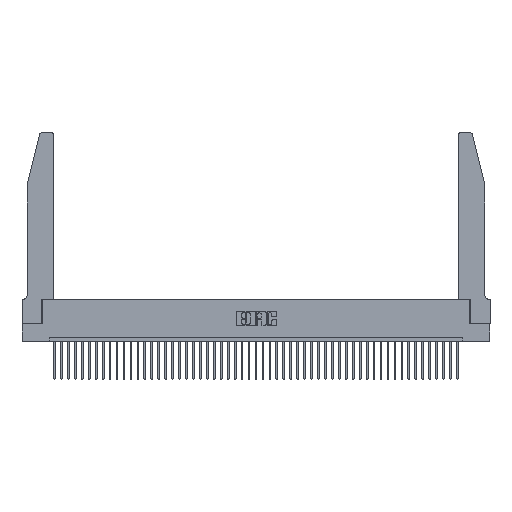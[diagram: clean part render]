
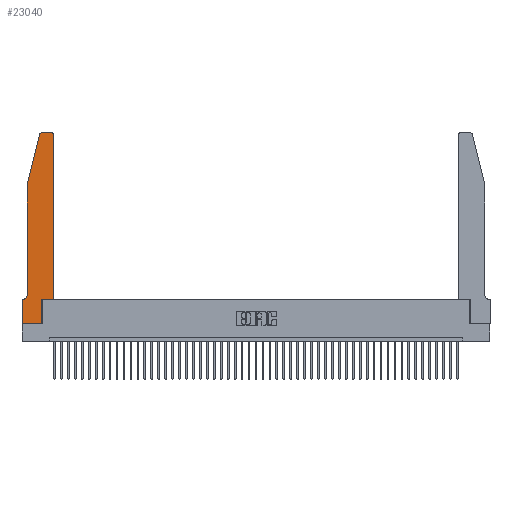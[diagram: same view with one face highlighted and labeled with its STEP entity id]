
A CAD part, top view. The second image highlights one B-rep face of the part: STEP entity #23040.
In plain terms, the highlighted planar face has unit normal (0, 0, 1).
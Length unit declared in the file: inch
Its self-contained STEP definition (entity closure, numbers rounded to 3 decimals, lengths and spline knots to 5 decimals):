
#337 = VECTOR ( 'NONE', #37796, 39.37008 ) ;
#1541 = EDGE_CURVE ( 'NONE', #1950, #15403, #41016, .T. ) ;
#1950 = VERTEX_POINT ( 'NONE', #6694 ) ;
#2095 = DIRECTION ( 'NONE',  ( -1., 0., 0. ) ) ;
#2553 = EDGE_CURVE ( 'NONE', #33714, #12018, #30086, .T. ) ;
#3229 = CARTESIAN_POINT ( 'NONE',  ( 0.0055, 0.42, 0.37 ) ) ;
#3548 = CARTESIAN_POINT ( 'NONE',  ( 0., 0.35, 0.37 ) ) ;
#3608 = CARTESIAN_POINT ( 'NONE',  ( 0., 0., 0.37 ) ) ;
#3663 = CARTESIAN_POINT ( 'NONE',  ( 0.2865, 0., 0.37 ) ) ;
#3755 = DIRECTION ( 'NONE',  ( 0., -1., 0. ) ) ;
#4073 = EDGE_CURVE ( 'NONE', #15403, #33714, #12669, .T. ) ;
#5394 = ORIENTED_EDGE ( 'NONE', *, *, #8380, .T. ) ;
#6399 = VECTOR ( 'NONE', #44380, 39.37008 ) ;
#6694 = CARTESIAN_POINT ( 'NONE',  ( 0.0755, 0.42, 0.37 ) ) ;
#6964 = ORIENTED_EDGE ( 'NONE', *, *, #18924, .T. ) ;
#7111 = LINE ( 'NONE', #45307, #44422 ) ;
#7650 = EDGE_CURVE ( 'NONE', #44659, #1950, #43006, .T. ) ;
#7919 = VERTEX_POINT ( 'NONE', #3663 ) ;
#8361 = CARTESIAN_POINT ( 'NONE',  ( 0.4505, 2.72, 0.37 ) ) ;
#8380 = EDGE_CURVE ( 'NONE', #26817, #12183, #8868, .T. ) ;
#8701 = DIRECTION ( 'NONE',  ( -0.239, -0.971, 0. ) ) ;
#8712 = ORIENTED_EDGE ( 'NONE', *, *, #30683, .T. ) ;
#8868 = LINE ( 'NONE', #12478, #337 ) ;
#9598 = DIRECTION ( 'NONE',  ( 1., 0., 0. ) ) ;
#9616 = CARTESIAN_POINT ( 'NONE',  ( 0.0755, 0.35, 0.37 ) ) ;
#10459 = CIRCLE ( 'NONE', #32345, 0.03 ) ;
#10673 = CARTESIAN_POINT ( 'NONE',  ( 0.4205, 2.72, 0.37 ) ) ;
#10820 = DIRECTION ( 'NONE',  ( 0., 0., 1. ) ) ;
#10960 = EDGE_CURVE ( 'NONE', #12018, #7919, #43681, .T. ) ;
#11431 = DIRECTION ( 'NONE',  ( -1., 0., 0. ) ) ;
#12018 = VERTEX_POINT ( 'NONE', #31430 ) ;
#12183 = VERTEX_POINT ( 'NONE', #8361 ) ;
#12478 = CARTESIAN_POINT ( 'NONE',  ( 0.4505, 0.35, 0.37 ) ) ;
#12669 = LINE ( 'NONE', #9616, #13843 ) ;
#13051 = ORIENTED_EDGE ( 'NONE', *, *, #15172, .T. ) ;
#13300 = PLANE ( 'NONE',  #20709 ) ;
#13843 = VECTOR ( 'NONE', #2095, 39.37008 ) ;
#15172 = EDGE_CURVE ( 'NONE', #25580, #36501, #10459, .T. ) ;
#15403 = VERTEX_POINT ( 'NONE', #16053 ) ;
#15436 = LINE ( 'NONE', #32141, #31980 ) ;
#16053 = CARTESIAN_POINT ( 'NONE',  ( 0.0055, 0.35, 0.37 ) ) ;
#18842 = EDGE_LOOP ( 'NONE', ( #41561, #13051, #8712, #39670, #31578, #46272, #38452, #45195, #22746, #6964, #5394, #21310 ) ) ;
#18924 = EDGE_CURVE ( 'NONE', #26772, #26817, #15436, .T. ) ;
#19479 = CARTESIAN_POINT ( 'NONE',  ( 0., 0.35, 0.37 ) ) ;
#20709 = AXIS2_PLACEMENT_3D ( 'NONE', #3548, #35948, #24825 ) ;
#20877 = AXIS2_PLACEMENT_3D ( 'NONE', #3229, #25839, #11431 ) ;
#21310 = ORIENTED_EDGE ( 'NONE', *, *, #44666, .T. ) ;
#21894 = DIRECTION ( 'NONE',  ( -1., 0., 0. ) ) ;
#22272 = CARTESIAN_POINT ( 'NONE',  ( 0.4505, 0.35, 0.37 ) ) ;
#22746 = ORIENTED_EDGE ( 'NONE', *, *, #34009, .T. ) ;
#23040 = ADVANCED_FACE ( 'NONE', ( #31679 ), #13300, .T. ) ;
#23845 = CARTESIAN_POINT ( 'NONE',  ( 0.284, 2.72, 0.37 ) ) ;
#24825 = DIRECTION ( 'NONE',  ( 1., 0., 0. ) ) ;
#25190 = LINE ( 'NONE', #40761, #6399 ) ;
#25580 = VERTEX_POINT ( 'NONE', #41471 ) ;
#25839 = DIRECTION ( 'NONE',  ( 0., 0., -1. ) ) ;
#26772 = VERTEX_POINT ( 'NONE', #44590 ) ;
#26817 = VERTEX_POINT ( 'NONE', #22272 ) ;
#27314 = CARTESIAN_POINT ( 'NONE',  ( 0.0755, 2., 0.37 ) ) ;
#29006 = VECTOR ( 'NONE', #3755, 39.37008 ) ;
#29299 = CARTESIAN_POINT ( 'NONE',  ( 0., 0., 0.37 ) ) ;
#29350 = VECTOR ( 'NONE', #45357, 39.37008 ) ;
#29370 = CIRCLE ( 'NONE', #46290, 0.03 ) ;
#30086 = LINE ( 'NONE', #3608, #29006 ) ;
#30683 = EDGE_CURVE ( 'NONE', #36501, #44659, #7111, .T. ) ;
#31288 = DIRECTION ( 'NONE',  ( 0., 0., 1. ) ) ;
#31430 = CARTESIAN_POINT ( 'NONE',  ( 0., 0., 0.37 ) ) ;
#31578 = ORIENTED_EDGE ( 'NONE', *, *, #1541, .T. ) ;
#31679 = FACE_OUTER_BOUND ( 'NONE', #18842, .T. ) ;
#31980 = VECTOR ( 'NONE', #39440, 39.37008 ) ;
#32141 = CARTESIAN_POINT ( 'NONE',  ( 0.4505, 0.35, 0.37 ) ) ;
#32345 = AXIS2_PLACEMENT_3D ( 'NONE', #23845, #31288, #9598 ) ;
#32822 = DIRECTION ( 'NONE',  ( 1., 0., 0. ) ) ;
#33714 = VERTEX_POINT ( 'NONE', #19479 ) ;
#34009 = EDGE_CURVE ( 'NONE', #7919, #26772, #25190, .T. ) ;
#34426 = CARTESIAN_POINT ( 'NONE',  ( 0.4205, 2.75, 0.37 ) ) ;
#34768 = CARTESIAN_POINT ( 'NONE',  ( 0.0755, 2., 0.37 ) ) ;
#35948 = DIRECTION ( 'NONE',  ( 0., 0., 1. ) ) ;
#36181 = DIRECTION ( 'NONE',  ( 1., 0., 0. ) ) ;
#36365 = VECTOR ( 'NONE', #32822, 39.37008 ) ;
#36501 = VERTEX_POINT ( 'NONE', #43581 ) ;
#37796 = DIRECTION ( 'NONE',  ( 0., 1., 0. ) ) ;
#38452 = ORIENTED_EDGE ( 'NONE', *, *, #2553, .T. ) ;
#39440 = DIRECTION ( 'NONE',  ( 1., 0., 0. ) ) ;
#39670 = ORIENTED_EDGE ( 'NONE', *, *, #7650, .T. ) ;
#40052 = LINE ( 'NONE', #43598, #40559 ) ;
#40559 = VECTOR ( 'NONE', #21894, 39.37008 ) ;
#40761 = CARTESIAN_POINT ( 'NONE',  ( 0.2865, 0.35, 0.37 ) ) ;
#41016 = CIRCLE ( 'NONE', #20877, 0.07 ) ;
#41471 = CARTESIAN_POINT ( 'NONE',  ( 0.284, 2.75, 0.37 ) ) ;
#41552 = VERTEX_POINT ( 'NONE', #34426 ) ;
#41561 = ORIENTED_EDGE ( 'NONE', *, *, #46041, .T. ) ;
#43006 = LINE ( 'NONE', #34768, #29350 ) ;
#43581 = CARTESIAN_POINT ( 'NONE',  ( 0.25487, 2.72718, 0.37 ) ) ;
#43598 = CARTESIAN_POINT ( 'NONE',  ( 0.2605, 2.75, 0.37 ) ) ;
#43681 = LINE ( 'NONE', #29299, #36365 ) ;
#44380 = DIRECTION ( 'NONE',  ( 0., 1., 0. ) ) ;
#44422 = VECTOR ( 'NONE', #8701, 39.37008 ) ;
#44590 = CARTESIAN_POINT ( 'NONE',  ( 0.2865, 0.35, 0.37 ) ) ;
#44659 = VERTEX_POINT ( 'NONE', #27314 ) ;
#44666 = EDGE_CURVE ( 'NONE', #12183, #41552, #29370, .T. ) ;
#45195 = ORIENTED_EDGE ( 'NONE', *, *, #10960, .T. ) ;
#45307 = CARTESIAN_POINT ( 'NONE',  ( 0.0755, 2., 0.37 ) ) ;
#45357 = DIRECTION ( 'NONE',  ( 0., -1., 0. ) ) ;
#46041 = EDGE_CURVE ( 'NONE', #41552, #25580, #40052, .T. ) ;
#46272 = ORIENTED_EDGE ( 'NONE', *, *, #4073, .T. ) ;
#46290 = AXIS2_PLACEMENT_3D ( 'NONE', #10673, #10820, #36181 ) ;
